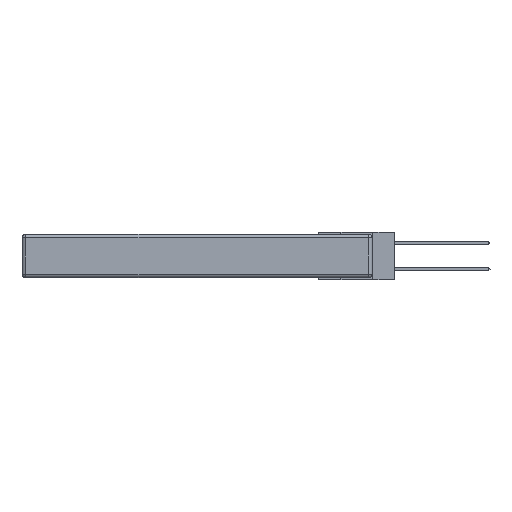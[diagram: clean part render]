
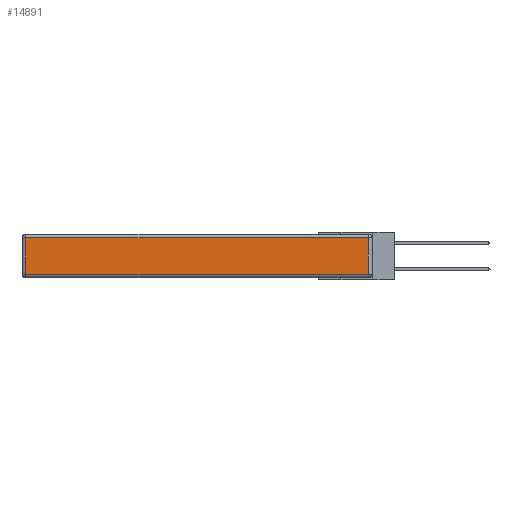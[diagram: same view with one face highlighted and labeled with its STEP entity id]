
A CAD part, left-side view. The second image highlights one B-rep face of the part: STEP entity #14891.
In plain terms, the highlighted planar face has unit normal (-1, 0, 0).
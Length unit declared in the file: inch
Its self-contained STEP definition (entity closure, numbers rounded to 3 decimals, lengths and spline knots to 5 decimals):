
#35 = LINE ( 'NONE', #13509, #15289 ) ;
#399 = CARTESIAN_POINT ( 'NONE',  ( 0., 2.72, -0.03 ) ) ;
#856 = PLANE ( 'NONE',  #17243 ) ;
#1246 = EDGE_CURVE ( 'NONE', #13800, #14240, #17447, .T. ) ;
#1751 = EDGE_CURVE ( 'NONE', #6487, #17412, #7269, .T. ) ;
#3017 = ORIENTED_EDGE ( 'NONE', *, *, #14120, .T. ) ;
#4663 = CARTESIAN_POINT ( 'NONE',  ( 0., 0., -0.313 ) ) ;
#6487 = VERTEX_POINT ( 'NONE', #8702 ) ;
#6509 = CARTESIAN_POINT ( 'NONE',  ( 0., 2.75, -0.03 ) ) ;
#6540 = EDGE_LOOP ( 'NONE', ( #16854, #14653, #9242, #3017 ) ) ;
#6636 = DIRECTION ( 'NONE',  ( 0., 1., 0. ) ) ;
#6842 = DIRECTION ( 'NONE',  ( 0., 0., 1. ) ) ;
#7269 = LINE ( 'NONE', #6509, #14640 ) ;
#7685 = EDGE_CURVE ( 'NONE', #14240, #6487, #18760, .T. ) ;
#8702 = CARTESIAN_POINT ( 'NONE',  ( 0., 0.03, -0.03 ) ) ;
#9242 = ORIENTED_EDGE ( 'NONE', *, *, #1751, .T. ) ;
#9461 = FACE_OUTER_BOUND ( 'NONE', #6540, .T. ) ;
#9782 = DIRECTION ( 'NONE',  ( 0., 0., 1. ) ) ;
#12154 = DIRECTION ( 'NONE',  ( 0., -1., 0. ) ) ;
#13185 = VECTOR ( 'NONE', #9782, 39.37008 ) ;
#13509 = CARTESIAN_POINT ( 'NONE',  ( 0., 2.72, -0.343 ) ) ;
#13800 = VERTEX_POINT ( 'NONE', #18425 ) ;
#14120 = EDGE_CURVE ( 'NONE', #17412, #13800, #35, .T. ) ;
#14240 = VERTEX_POINT ( 'NONE', #18573 ) ;
#14640 = VECTOR ( 'NONE', #6636, 39.37008 ) ;
#14653 = ORIENTED_EDGE ( 'NONE', *, *, #7685, .T. ) ;
#14891 = ADVANCED_FACE ( 'NONE', ( #9461 ), #856, .T. ) ;
#15142 = DIRECTION ( 'NONE',  ( 0., 0., -1. ) ) ;
#15156 = VECTOR ( 'NONE', #12154, 39.37008 ) ;
#15224 = CARTESIAN_POINT ( 'NONE',  ( 0., 0.03, -0.343 ) ) ;
#15289 = VECTOR ( 'NONE', #15142, 39.37008 ) ;
#16854 = ORIENTED_EDGE ( 'NONE', *, *, #1246, .T. ) ;
#17239 = CARTESIAN_POINT ( 'NONE',  ( 0., 0., -0.343 ) ) ;
#17243 = AXIS2_PLACEMENT_3D ( 'NONE', #17239, #18680, #6842 ) ;
#17412 = VERTEX_POINT ( 'NONE', #399 ) ;
#17447 = LINE ( 'NONE', #4663, #15156 ) ;
#18425 = CARTESIAN_POINT ( 'NONE',  ( 0., 2.72, -0.313 ) ) ;
#18573 = CARTESIAN_POINT ( 'NONE',  ( 0., 0.03, -0.313 ) ) ;
#18680 = DIRECTION ( 'NONE',  ( -1., 0., 0. ) ) ;
#18760 = LINE ( 'NONE', #15224, #13185 ) ;
